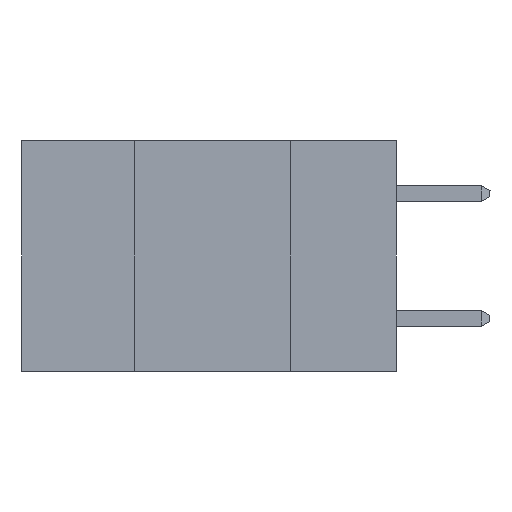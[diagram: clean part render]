
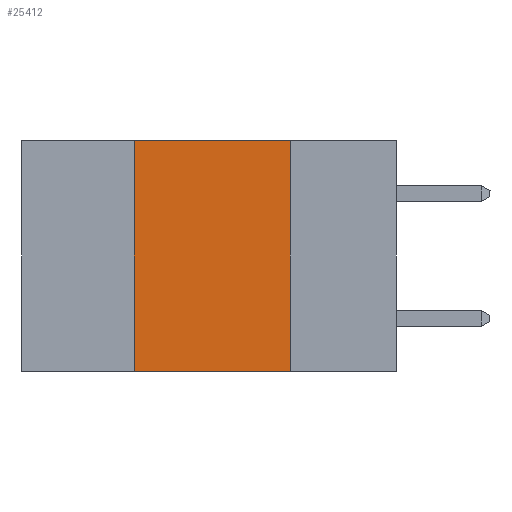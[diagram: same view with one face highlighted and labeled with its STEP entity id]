
A CAD part, left-side view. The second image highlights one B-rep face of the part: STEP entity #25412.
In plain terms, the highlighted planar face has unit normal (-1, 0, 0).
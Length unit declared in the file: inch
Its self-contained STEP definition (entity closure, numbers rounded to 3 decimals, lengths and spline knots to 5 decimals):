
#381 = VECTOR ( 'NONE', #17007, 39.37008 ) ;
#2129 = VERTEX_POINT ( 'NONE', #28341 ) ;
#2764 = EDGE_CURVE ( 'NONE', #23969, #2129, #19642, .T. ) ;
#6089 = PLANE ( 'NONE',  #25162 ) ;
#7503 = ORIENTED_EDGE ( 'NONE', *, *, #2764, .F. ) ;
#7940 = VECTOR ( 'NONE', #12131, 39.37008 ) ;
#8585 = DIRECTION ( 'NONE',  ( 0., 0., -1. ) ) ;
#8880 = EDGE_LOOP ( 'NONE', ( #10975, #7503, #25219, #30752 ) ) ;
#9303 = LINE ( 'NONE', #32037, #21856 ) ;
#9480 = DIRECTION ( 'NONE',  ( 0., 0., -1. ) ) ;
#9638 = CARTESIAN_POINT ( 'NONE',  ( 0., 0.6, -0.37 ) ) ;
#9764 = CARTESIAN_POINT ( 'NONE',  ( 0., 0.42, -0.37 ) ) ;
#10194 = VERTEX_POINT ( 'NONE', #11360 ) ;
#10497 = CARTESIAN_POINT ( 'NONE',  ( 0., 0.42, 0. ) ) ;
#10975 = ORIENTED_EDGE ( 'NONE', *, *, #27581, .F. ) ;
#11154 = LINE ( 'NONE', #10497, #28901 ) ;
#11360 = CARTESIAN_POINT ( 'NONE',  ( 0., 0.17, -0.37 ) ) ;
#12131 = DIRECTION ( 'NONE',  ( 0., -1., 0. ) ) ;
#13004 = DIRECTION ( 'NONE',  ( 0., 0., 1. ) ) ;
#13117 = VERTEX_POINT ( 'NONE', #9764 ) ;
#17007 = DIRECTION ( 'NONE',  ( 0., -1., 0. ) ) ;
#19642 = LINE ( 'NONE', #25243, #381 ) ;
#20755 = EDGE_CURVE ( 'NONE', #13117, #10194, #21255, .T. ) ;
#20907 = FACE_OUTER_BOUND ( 'NONE', #8880, .T. ) ;
#21255 = LINE ( 'NONE', #9638, #7940 ) ;
#21856 = VECTOR ( 'NONE', #9480, 39.37008 ) ;
#23526 = CARTESIAN_POINT ( 'NONE',  ( 0., 0.6, 0. ) ) ;
#23632 = DIRECTION ( 'NONE',  ( 1., 0., 0. ) ) ;
#23969 = VERTEX_POINT ( 'NONE', #27760 ) ;
#25162 = AXIS2_PLACEMENT_3D ( 'NONE', #23526, #23632, #8585 ) ;
#25219 = ORIENTED_EDGE ( 'NONE', *, *, #28620, .F. ) ;
#25243 = CARTESIAN_POINT ( 'NONE',  ( 0., 0.6, 0. ) ) ;
#25412 = ADVANCED_FACE ( 'NONE', ( #20907 ), #6089, .F. ) ;
#27581 = EDGE_CURVE ( 'NONE', #2129, #10194, #9303, .T. ) ;
#27760 = CARTESIAN_POINT ( 'NONE',  ( 0., 0.42, 0. ) ) ;
#28341 = CARTESIAN_POINT ( 'NONE',  ( 0., 0.17, 0. ) ) ;
#28620 = EDGE_CURVE ( 'NONE', #13117, #23969, #11154, .T. ) ;
#28901 = VECTOR ( 'NONE', #13004, 39.37008 ) ;
#30752 = ORIENTED_EDGE ( 'NONE', *, *, #20755, .T. ) ;
#32037 = CARTESIAN_POINT ( 'NONE',  ( 0., 0.17, 0. ) ) ;
